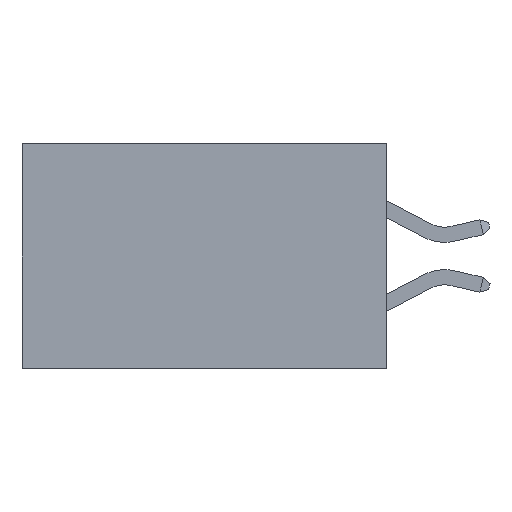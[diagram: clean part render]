
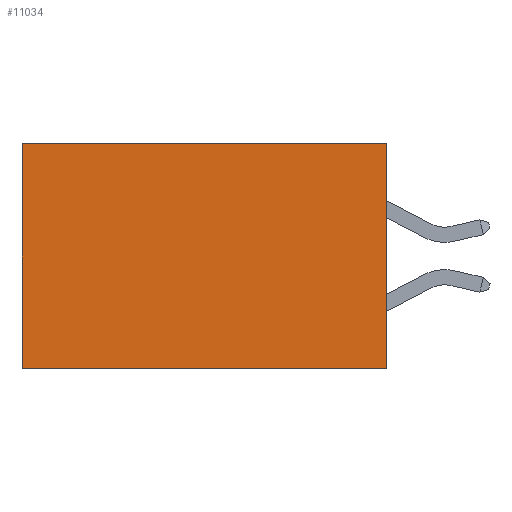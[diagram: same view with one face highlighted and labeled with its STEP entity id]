
A CAD part, left-side view. The second image highlights one B-rep face of the part: STEP entity #11034.
In plain terms, the highlighted planar face has unit normal (-1, 0, 0).
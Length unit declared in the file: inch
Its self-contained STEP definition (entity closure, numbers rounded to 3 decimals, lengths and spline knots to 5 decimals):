
#345 = EDGE_CURVE ( 'NONE', #4351, #967, #2864, .T. ) ;
#504 = VECTOR ( 'NONE', #4312, 39.37008 ) ;
#701 = CARTESIAN_POINT ( 'NONE',  ( 0.2615, 0., -0.37 ) ) ;
#782 = DIRECTION ( 'NONE',  ( 0., 1., 0. ) ) ;
#967 = VERTEX_POINT ( 'NONE', #1212 ) ;
#1212 = CARTESIAN_POINT ( 'NONE',  ( 0.2615, 0., -0.37 ) ) ;
#1777 = EDGE_CURVE ( 'NONE', #4351, #3745, #5023, .T. ) ;
#1965 = PLANE ( 'NONE',  #4573 ) ;
#2864 = LINE ( 'NONE', #7425, #504 ) ;
#2973 = DIRECTION ( 'NONE',  ( 1., 0., 0. ) ) ;
#3249 = VECTOR ( 'NONE', #9857, 39.37008 ) ;
#3675 = EDGE_CURVE ( 'NONE', #967, #8032, #8496, .T. ) ;
#3745 = VERTEX_POINT ( 'NONE', #12918 ) ;
#4098 = ORIENTED_EDGE ( 'NONE', *, *, #345, .F. ) ;
#4312 = DIRECTION ( 'NONE',  ( 0., 0., -1. ) ) ;
#4351 = VERTEX_POINT ( 'NONE', #9860 ) ;
#4573 = AXIS2_PLACEMENT_3D ( 'NONE', #9102, #2973, #10099 ) ;
#5023 = LINE ( 'NONE', #11230, #7457 ) ;
#5917 = EDGE_LOOP ( 'NONE', ( #9547, #9290, #4098, #8970 ) ) ;
#6309 = LINE ( 'NONE', #6805, #3249 ) ;
#6805 = CARTESIAN_POINT ( 'NONE',  ( 0.2615, 0.6, -0.37 ) ) ;
#6885 = CARTESIAN_POINT ( 'NONE',  ( 0.2615, 0.6, -0.37 ) ) ;
#7190 = FACE_OUTER_BOUND ( 'NONE', #5917, .T. ) ;
#7425 = CARTESIAN_POINT ( 'NONE',  ( 0.2615, 0., -0.37 ) ) ;
#7457 = VECTOR ( 'NONE', #11082, 39.37008 ) ;
#7978 = EDGE_CURVE ( 'NONE', #3745, #8032, #6309, .T. ) ;
#8032 = VERTEX_POINT ( 'NONE', #6885 ) ;
#8179 = VECTOR ( 'NONE', #782, 39.37008 ) ;
#8496 = LINE ( 'NONE', #701, #8179 ) ;
#8970 = ORIENTED_EDGE ( 'NONE', *, *, #1777, .T. ) ;
#9102 = CARTESIAN_POINT ( 'NONE',  ( 0.2615, 0., -0.37 ) ) ;
#9290 = ORIENTED_EDGE ( 'NONE', *, *, #3675, .F. ) ;
#9547 = ORIENTED_EDGE ( 'NONE', *, *, #7978, .T. ) ;
#9857 = DIRECTION ( 'NONE',  ( 0., 0., -1. ) ) ;
#9860 = CARTESIAN_POINT ( 'NONE',  ( 0.2615, 0., 0. ) ) ;
#10099 = DIRECTION ( 'NONE',  ( 0., 0., -1. ) ) ;
#11034 = ADVANCED_FACE ( 'NONE', ( #7190 ), #1965, .F. ) ;
#11082 = DIRECTION ( 'NONE',  ( 0., 1., 0. ) ) ;
#11230 = CARTESIAN_POINT ( 'NONE',  ( 0.2615, 0., 0. ) ) ;
#12918 = CARTESIAN_POINT ( 'NONE',  ( 0.2615, 0.6, 0. ) ) ;
